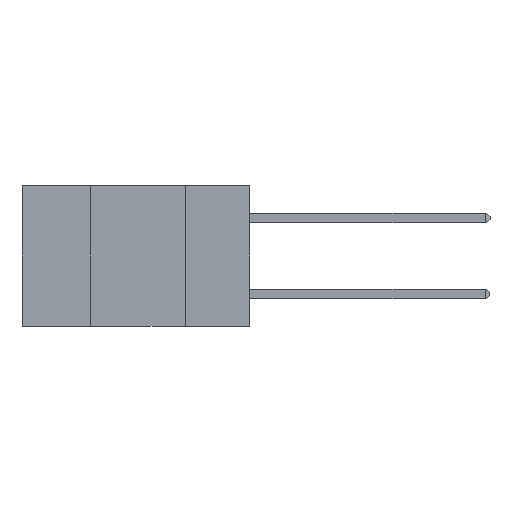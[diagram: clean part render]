
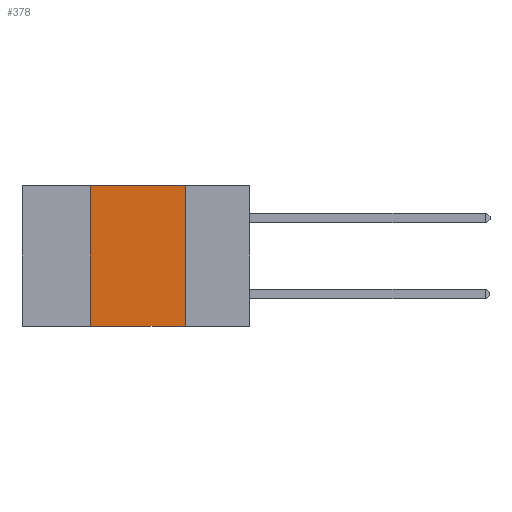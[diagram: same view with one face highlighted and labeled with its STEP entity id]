
A CAD part, left-side view. The second image highlights one B-rep face of the part: STEP entity #378.
In plain terms, the highlighted planar face has unit normal (-1, 0, 0).
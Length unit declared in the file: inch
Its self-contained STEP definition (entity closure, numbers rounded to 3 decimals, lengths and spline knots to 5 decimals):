
#77 = VECTOR ( 'NONE', #2802, 39.37008 ) ;
#378 = ADVANCED_FACE ( 'NONE', ( #1077 ), #5795, .F. ) ;
#657 = VERTEX_POINT ( 'NONE', #3779 ) ;
#778 = EDGE_CURVE ( 'NONE', #3262, #6807, #4529, .T. ) ;
#827 = VERTEX_POINT ( 'NONE', #2477 ) ;
#1077 = FACE_OUTER_BOUND ( 'NONE', #6173, .T. ) ;
#1099 = AXIS2_PLACEMENT_3D ( 'NONE', #5920, #4997, #9463 ) ;
#1442 = CARTESIAN_POINT ( 'NONE',  ( 0., 0.6, 0. ) ) ;
#1735 = LINE ( 'NONE', #6122, #3667 ) ;
#2466 = DIRECTION ( 'NONE',  ( 0., 0., -1. ) ) ;
#2477 = CARTESIAN_POINT ( 'NONE',  ( 0., 0.17, -0.37 ) ) ;
#2665 = LINE ( 'NONE', #5660, #4580 ) ;
#2802 = DIRECTION ( 'NONE',  ( 0., -1., 0. ) ) ;
#2977 = DIRECTION ( 'NONE',  ( 0., 0., 1. ) ) ;
#3262 = VERTEX_POINT ( 'NONE', #5965 ) ;
#3667 = VECTOR ( 'NONE', #2977, 39.37008 ) ;
#3779 = CARTESIAN_POINT ( 'NONE',  ( 0., 0.42, -0.37 ) ) ;
#3925 = ORIENTED_EDGE ( 'NONE', *, *, #8627, .F. ) ;
#4066 = EDGE_CURVE ( 'NONE', #657, #827, #8087, .T. ) ;
#4219 = ORIENTED_EDGE ( 'NONE', *, *, #778, .F. ) ;
#4227 = ORIENTED_EDGE ( 'NONE', *, *, #4066, .T. ) ;
#4529 = LINE ( 'NONE', #1442, #77 ) ;
#4580 = VECTOR ( 'NONE', #2466, 39.37008 ) ;
#4997 = DIRECTION ( 'NONE',  ( 1., 0., 0. ) ) ;
#5123 = EDGE_CURVE ( 'NONE', #6807, #827, #2665, .T. ) ;
#5660 = CARTESIAN_POINT ( 'NONE',  ( 0., 0.17, 0. ) ) ;
#5795 = PLANE ( 'NONE',  #1099 ) ;
#5920 = CARTESIAN_POINT ( 'NONE',  ( 0., 0.6, 0. ) ) ;
#5965 = CARTESIAN_POINT ( 'NONE',  ( 0., 0.42, 0. ) ) ;
#6071 = CARTESIAN_POINT ( 'NONE',  ( 0., 0.6, -0.37 ) ) ;
#6108 = DIRECTION ( 'NONE',  ( 0., -1., 0. ) ) ;
#6122 = CARTESIAN_POINT ( 'NONE',  ( 0., 0.42, 0. ) ) ;
#6173 = EDGE_LOOP ( 'NONE', ( #6252, #4219, #3925, #4227 ) ) ;
#6241 = CARTESIAN_POINT ( 'NONE',  ( 0., 0.17, 0. ) ) ;
#6252 = ORIENTED_EDGE ( 'NONE', *, *, #5123, .F. ) ;
#6807 = VERTEX_POINT ( 'NONE', #6241 ) ;
#8087 = LINE ( 'NONE', #6071, #9351 ) ;
#8627 = EDGE_CURVE ( 'NONE', #657, #3262, #1735, .T. ) ;
#9351 = VECTOR ( 'NONE', #6108, 39.37008 ) ;
#9463 = DIRECTION ( 'NONE',  ( 0., 0., -1. ) ) ;
